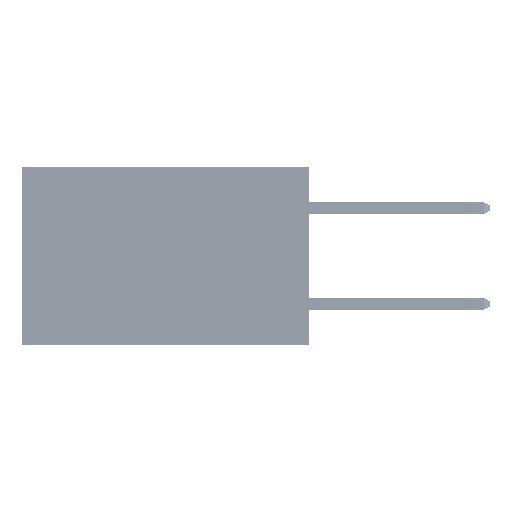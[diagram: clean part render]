
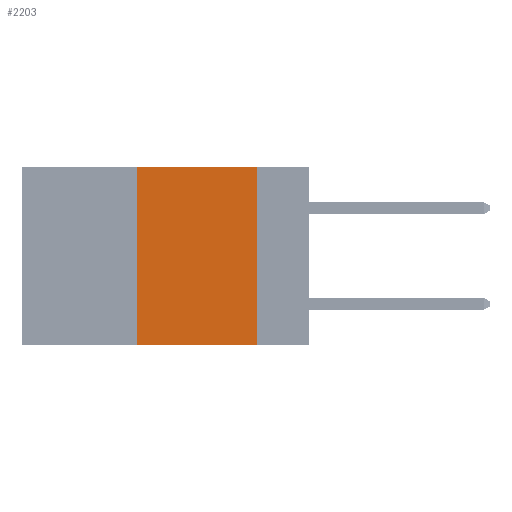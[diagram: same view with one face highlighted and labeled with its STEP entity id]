
A CAD part, left-side view. The second image highlights one B-rep face of the part: STEP entity #2203.
In plain terms, the highlighted planar face has unit normal (-1, 0, 0).
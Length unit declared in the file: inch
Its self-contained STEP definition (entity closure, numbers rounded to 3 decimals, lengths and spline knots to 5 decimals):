
#645 = DIRECTION ( 'NONE',  ( 0., 0., -1. ) ) ;
#2203 = ADVANCED_FACE ( 'NONE', ( #29394 ), #7283, .F. ) ;
#2570 = CARTESIAN_POINT ( 'NONE',  ( 0., 0.11, 0. ) ) ;
#5546 = VECTOR ( 'NONE', #9695, 39.37008 ) ;
#5834 = CARTESIAN_POINT ( 'NONE',  ( 0., 0.36, 0. ) ) ;
#7283 = PLANE ( 'NONE',  #7700 ) ;
#7700 = AXIS2_PLACEMENT_3D ( 'NONE', #10729, #37234, #25708 ) ;
#8052 = CARTESIAN_POINT ( 'NONE',  ( 0., 0.36, 0. ) ) ;
#8608 = CARTESIAN_POINT ( 'NONE',  ( 0., 0.11, -0.37 ) ) ;
#9695 = DIRECTION ( 'NONE',  ( 0., -1., 0. ) ) ;
#10729 = CARTESIAN_POINT ( 'NONE',  ( 0., 0.6, 0. ) ) ;
#11693 = VECTOR ( 'NONE', #645, 39.37008 ) ;
#14748 = ORIENTED_EDGE ( 'NONE', *, *, #27810, .T. ) ;
#14759 = EDGE_CURVE ( 'NONE', #32493, #45598, #46306, .T. ) ;
#15441 = LINE ( 'NONE', #8052, #21666 ) ;
#17030 = VECTOR ( 'NONE', #36193, 39.37008 ) ;
#18536 = CARTESIAN_POINT ( 'NONE',  ( 0., 0.36, -0.37 ) ) ;
#21666 = VECTOR ( 'NONE', #26727, 39.37008 ) ;
#23744 = ORIENTED_EDGE ( 'NONE', *, *, #14759, .F. ) ;
#24911 = LINE ( 'NONE', #46778, #5546 ) ;
#25708 = DIRECTION ( 'NONE',  ( 0., 0., -1. ) ) ;
#26727 = DIRECTION ( 'NONE',  ( 0., 0., 1. ) ) ;
#27810 = EDGE_CURVE ( 'NONE', #40276, #45598, #24911, .T. ) ;
#29061 = ORIENTED_EDGE ( 'NONE', *, *, #42996, .F. ) ;
#29078 = LINE ( 'NONE', #47258, #17030 ) ;
#29394 = FACE_OUTER_BOUND ( 'NONE', #35587, .T. ) ;
#32493 = VERTEX_POINT ( 'NONE', #2570 ) ;
#33359 = VERTEX_POINT ( 'NONE', #5834 ) ;
#35587 = EDGE_LOOP ( 'NONE', ( #23744, #47946, #29061, #14748 ) ) ;
#36193 = DIRECTION ( 'NONE',  ( 0., -1., 0. ) ) ;
#37234 = DIRECTION ( 'NONE',  ( 1., 0., 0. ) ) ;
#40276 = VERTEX_POINT ( 'NONE', #18536 ) ;
#42996 = EDGE_CURVE ( 'NONE', #40276, #33359, #15441, .T. ) ;
#43681 = EDGE_CURVE ( 'NONE', #33359, #32493, #29078, .T. ) ;
#45598 = VERTEX_POINT ( 'NONE', #8608 ) ;
#46064 = CARTESIAN_POINT ( 'NONE',  ( 0., 0.11, 0. ) ) ;
#46306 = LINE ( 'NONE', #46064, #11693 ) ;
#46778 = CARTESIAN_POINT ( 'NONE',  ( 0., 0.6, -0.37 ) ) ;
#47258 = CARTESIAN_POINT ( 'NONE',  ( 0., 0.6, 0. ) ) ;
#47946 = ORIENTED_EDGE ( 'NONE', *, *, #43681, .F. ) ;
